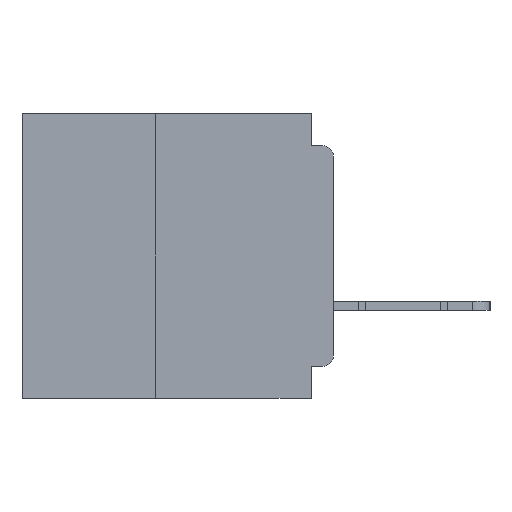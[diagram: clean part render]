
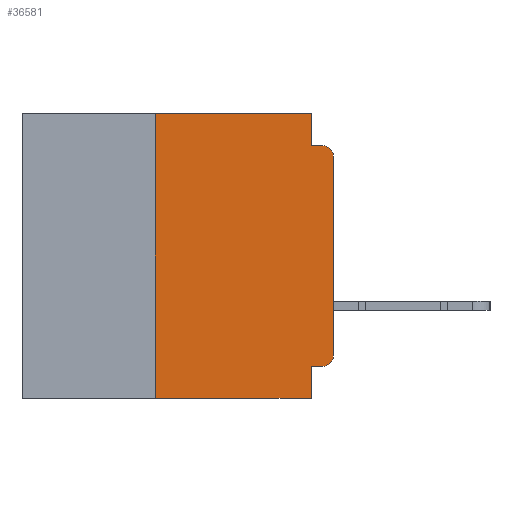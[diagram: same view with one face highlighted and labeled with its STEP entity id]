
A CAD part, left-side view. The second image highlights one B-rep face of the part: STEP entity #36581.
In plain terms, the highlighted planar face has unit normal (-1, 0, 0).
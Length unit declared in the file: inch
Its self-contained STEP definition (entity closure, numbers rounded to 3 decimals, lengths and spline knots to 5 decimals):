
#502 = LINE ( 'NONE', #64908, #64565 ) ;
#2981 = EDGE_LOOP ( 'NONE', ( #7161, #8738, #40380, #3218, #34872, #23046, #24592, #42802, #22285, #10397 ) ) ;
#2982 = CARTESIAN_POINT ( 'NONE',  ( 0., 0.25, 0. ) ) ;
#3218 = ORIENTED_EDGE ( 'NONE', *, *, #7138, .F. ) ;
#4874 = EDGE_CURVE ( 'NONE', #47245, #28260, #8701, .T. ) ;
#5365 = EDGE_CURVE ( 'NONE', #47260, #28260, #18950, .T. ) ;
#7138 = EDGE_CURVE ( 'NONE', #21041, #47260, #30575, .T. ) ;
#7161 = ORIENTED_EDGE ( 'NONE', *, *, #28287, .T. ) ;
#8006 = DIRECTION ( 'NONE',  ( 0., -1., 0. ) ) ;
#8701 = CIRCLE ( 'NONE', #12985, 0.015 ) ;
#8738 = ORIENTED_EDGE ( 'NONE', *, *, #4874, .T. ) ;
#10397 = ORIENTED_EDGE ( 'NONE', *, *, #18329, .T. ) ;
#12985 = AXIS2_PLACEMENT_3D ( 'NONE', #48678, #18480, #53793 ) ;
#13119 = PLANE ( 'NONE',  #20278 ) ;
#13624 = CARTESIAN_POINT ( 'NONE',  ( 0., 0.031, 0. ) ) ;
#13764 = VECTOR ( 'NONE', #24345, 39.37008 ) ;
#14296 = EDGE_CURVE ( 'NONE', #33599, #21041, #59088, .T. ) ;
#16261 = CARTESIAN_POINT ( 'NONE',  ( 0., 0., 0. ) ) ;
#18329 = EDGE_CURVE ( 'NONE', #34423, #52063, #23504, .T. ) ;
#18480 = DIRECTION ( 'NONE',  ( -1., 0., 0. ) ) ;
#18950 = LINE ( 'NONE', #33248, #44199 ) ;
#19056 = CARTESIAN_POINT ( 'NONE',  ( 0., 0., -0.355 ) ) ;
#19448 = DIRECTION ( 'NONE',  ( 0., -1., 0. ) ) ;
#20185 = CARTESIAN_POINT ( 'NONE',  ( 0., 0.437, 0. ) ) ;
#20278 = AXIS2_PLACEMENT_3D ( 'NONE', #43341, #28354, #63663 ) ;
#20540 = CARTESIAN_POINT ( 'NONE',  ( 0., 0.031, -0.4 ) ) ;
#21041 = VERTEX_POINT ( 'NONE', #13624 ) ;
#21319 = DIRECTION ( 'NONE',  ( 0., 0., 1. ) ) ;
#21484 = EDGE_CURVE ( 'NONE', #34423, #47860, #59480, .T. ) ;
#22285 = ORIENTED_EDGE ( 'NONE', *, *, #21484, .F. ) ;
#23046 = ORIENTED_EDGE ( 'NONE', *, *, #41600, .F. ) ;
#23148 = CARTESIAN_POINT ( 'NONE',  ( 0., 0.031, -0.355 ) ) ;
#23504 = CIRCLE ( 'NONE', #43449, 0.015 ) ;
#23979 = VERTEX_POINT ( 'NONE', #20540 ) ;
#24134 = DIRECTION ( 'NONE',  ( 0., 1., 0. ) ) ;
#24201 = DIRECTION ( 'NONE',  ( -1., 0., 0. ) ) ;
#24345 = DIRECTION ( 'NONE',  ( 0., 0., 1. ) ) ;
#24592 = ORIENTED_EDGE ( 'NONE', *, *, #63384, .T. ) ;
#26247 = DIRECTION ( 'NONE',  ( 0., 0., -1. ) ) ;
#28260 = VERTEX_POINT ( 'NONE', #51127 ) ;
#28287 = EDGE_CURVE ( 'NONE', #52063, #47245, #31089, .T. ) ;
#28354 = DIRECTION ( 'NONE',  ( 1., 0., 0. ) ) ;
#30575 = LINE ( 'NONE', #46879, #42408 ) ;
#31089 = LINE ( 'NONE', #16261, #56330 ) ;
#32276 = VECTOR ( 'NONE', #35195, 39.37008 ) ;
#32681 = VECTOR ( 'NONE', #24134, 39.37008 ) ;
#33248 = CARTESIAN_POINT ( 'NONE',  ( 0., 0., -0.045 ) ) ;
#33599 = VERTEX_POINT ( 'NONE', #2982 ) ;
#34423 = VERTEX_POINT ( 'NONE', #40416 ) ;
#34872 = ORIENTED_EDGE ( 'NONE', *, *, #14296, .F. ) ;
#35195 = DIRECTION ( 'NONE',  ( 0., -1., 0. ) ) ;
#35913 = CARTESIAN_POINT ( 'NONE',  ( 0., 0., -0.34 ) ) ;
#36581 = ADVANCED_FACE ( 'NONE', ( #64428 ), #13119, .F. ) ;
#39049 = LINE ( 'NONE', #59680, #13764 ) ;
#40242 = CARTESIAN_POINT ( 'NONE',  ( 0., 0.25, -0.4 ) ) ;
#40380 = ORIENTED_EDGE ( 'NONE', *, *, #5365, .F. ) ;
#40416 = CARTESIAN_POINT ( 'NONE',  ( 0., 0.015, -0.355 ) ) ;
#41274 = CARTESIAN_POINT ( 'NONE',  ( 0., 0.031, -0.4 ) ) ;
#41600 = EDGE_CURVE ( 'NONE', #41739, #33599, #39049, .T. ) ;
#41714 = VECTOR ( 'NONE', #26247, 39.37008 ) ;
#41739 = VERTEX_POINT ( 'NONE', #40242 ) ;
#42408 = VECTOR ( 'NONE', #47112, 39.37008 ) ;
#42802 = ORIENTED_EDGE ( 'NONE', *, *, #57201, .F. ) ;
#43341 = CARTESIAN_POINT ( 'NONE',  ( 0., 0.437, 0. ) ) ;
#43449 = AXIS2_PLACEMENT_3D ( 'NONE', #54465, #24201, #59531 ) ;
#44199 = VECTOR ( 'NONE', #8006, 39.37008 ) ;
#46879 = CARTESIAN_POINT ( 'NONE',  ( 0., 0.031, 0. ) ) ;
#47112 = DIRECTION ( 'NONE',  ( 0., 0., -1. ) ) ;
#47245 = VERTEX_POINT ( 'NONE', #58111 ) ;
#47260 = VERTEX_POINT ( 'NONE', #48350 ) ;
#47860 = VERTEX_POINT ( 'NONE', #23148 ) ;
#48350 = CARTESIAN_POINT ( 'NONE',  ( 0., 0.031, -0.045 ) ) ;
#48678 = CARTESIAN_POINT ( 'NONE',  ( 0., 0.015, -0.06 ) ) ;
#51127 = CARTESIAN_POINT ( 'NONE',  ( 0., 0.015, -0.045 ) ) ;
#52063 = VERTEX_POINT ( 'NONE', #35913 ) ;
#53793 = DIRECTION ( 'NONE',  ( 0., 0., -1. ) ) ;
#54465 = CARTESIAN_POINT ( 'NONE',  ( 0., 0.015, -0.34 ) ) ;
#55139 = LINE ( 'NONE', #41274, #41714 ) ;
#56330 = VECTOR ( 'NONE', #21319, 39.37008 ) ;
#57201 = EDGE_CURVE ( 'NONE', #47860, #23979, #55139, .T. ) ;
#58111 = CARTESIAN_POINT ( 'NONE',  ( 0., 0., -0.06 ) ) ;
#59088 = LINE ( 'NONE', #20185, #32276 ) ;
#59480 = LINE ( 'NONE', #19056, #32681 ) ;
#59531 = DIRECTION ( 'NONE',  ( 0., 0., -1. ) ) ;
#59680 = CARTESIAN_POINT ( 'NONE',  ( 0., 0.25, -0.4 ) ) ;
#63384 = EDGE_CURVE ( 'NONE', #41739, #23979, #502, .T. ) ;
#63663 = DIRECTION ( 'NONE',  ( 0., 0., -1. ) ) ;
#64428 = FACE_OUTER_BOUND ( 'NONE', #2981, .T. ) ;
#64565 = VECTOR ( 'NONE', #19448, 39.37008 ) ;
#64908 = CARTESIAN_POINT ( 'NONE',  ( 0., 0.437, -0.4 ) ) ;
